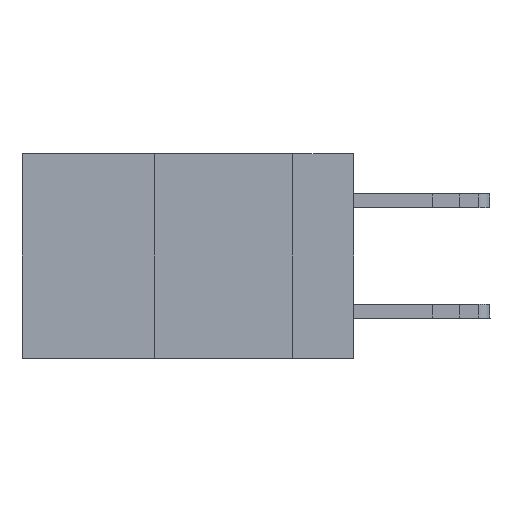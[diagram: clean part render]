
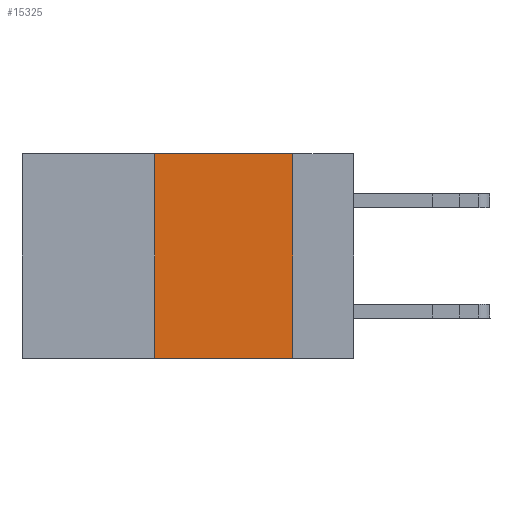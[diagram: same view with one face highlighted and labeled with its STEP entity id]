
A CAD part, left-side view. The second image highlights one B-rep face of the part: STEP entity #15325.
In plain terms, the highlighted planar face has unit normal (-1, 0, 0).
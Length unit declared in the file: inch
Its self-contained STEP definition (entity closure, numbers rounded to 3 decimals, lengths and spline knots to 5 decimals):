
#613 = ORIENTED_EDGE ( 'NONE', *, *, #15180, .F. ) ;
#630 = CARTESIAN_POINT ( 'NONE',  ( 0., 0.11, 0. ) ) ;
#675 = CARTESIAN_POINT ( 'NONE',  ( 0., 0.36, 0. ) ) ;
#763 = VERTEX_POINT ( 'NONE', #18695 ) ;
#1093 = CARTESIAN_POINT ( 'NONE',  ( 0., 0.6, 0. ) ) ;
#1596 = VERTEX_POINT ( 'NONE', #18190 ) ;
#1704 = DIRECTION ( 'NONE',  ( 0., -1., 0. ) ) ;
#1825 = VECTOR ( 'NONE', #3878, 39.37008 ) ;
#3130 = VECTOR ( 'NONE', #1704, 39.37008 ) ;
#3878 = DIRECTION ( 'NONE',  ( 0., -1., 0. ) ) ;
#4100 = DIRECTION ( 'NONE',  ( 0., 0., 1. ) ) ;
#5561 = VECTOR ( 'NONE', #4100, 39.37008 ) ;
#6224 = DIRECTION ( 'NONE',  ( 1., 0., 0. ) ) ;
#6231 = ORIENTED_EDGE ( 'NONE', *, *, #19114, .T. ) ;
#6248 = LINE ( 'NONE', #630, #14220 ) ;
#7597 = VERTEX_POINT ( 'NONE', #10774 ) ;
#8268 = EDGE_CURVE ( 'NONE', #763, #11267, #19087, .T. ) ;
#9611 = ORIENTED_EDGE ( 'NONE', *, *, #8268, .F. ) ;
#9818 = EDGE_LOOP ( 'NONE', ( #613, #18676, #9611, #6231 ) ) ;
#10774 = CARTESIAN_POINT ( 'NONE',  ( 0., 0.11, -0.37 ) ) ;
#10976 = CARTESIAN_POINT ( 'NONE',  ( 0., 0.36, 0. ) ) ;
#11267 = VERTEX_POINT ( 'NONE', #10976 ) ;
#11567 = LINE ( 'NONE', #15301, #3130 ) ;
#12612 = DIRECTION ( 'NONE',  ( 0., 0., -1. ) ) ;
#14004 = EDGE_CURVE ( 'NONE', #11267, #1596, #11567, .T. ) ;
#14220 = VECTOR ( 'NONE', #12612, 39.37008 ) ;
#15077 = AXIS2_PLACEMENT_3D ( 'NONE', #1093, #6224, #18055 ) ;
#15180 = EDGE_CURVE ( 'NONE', #1596, #7597, #6248, .T. ) ;
#15301 = CARTESIAN_POINT ( 'NONE',  ( 0., 0.6, 0. ) ) ;
#15325 = ADVANCED_FACE ( 'NONE', ( #21468 ), #16389, .F. ) ;
#16389 = PLANE ( 'NONE',  #15077 ) ;
#18055 = DIRECTION ( 'NONE',  ( 0., 0., -1. ) ) ;
#18190 = CARTESIAN_POINT ( 'NONE',  ( 0., 0.11, 0. ) ) ;
#18676 = ORIENTED_EDGE ( 'NONE', *, *, #14004, .F. ) ;
#18695 = CARTESIAN_POINT ( 'NONE',  ( 0., 0.36, -0.37 ) ) ;
#19057 = CARTESIAN_POINT ( 'NONE',  ( 0., 0.6, -0.37 ) ) ;
#19087 = LINE ( 'NONE', #675, #5561 ) ;
#19114 = EDGE_CURVE ( 'NONE', #763, #7597, #19811, .T. ) ;
#19811 = LINE ( 'NONE', #19057, #1825 ) ;
#21468 = FACE_OUTER_BOUND ( 'NONE', #9818, .T. ) ;
